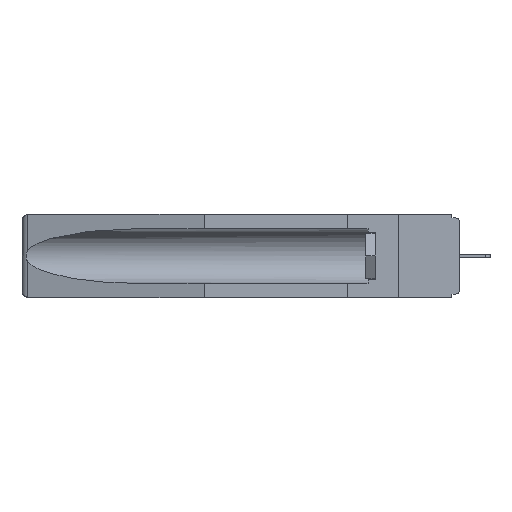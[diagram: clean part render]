
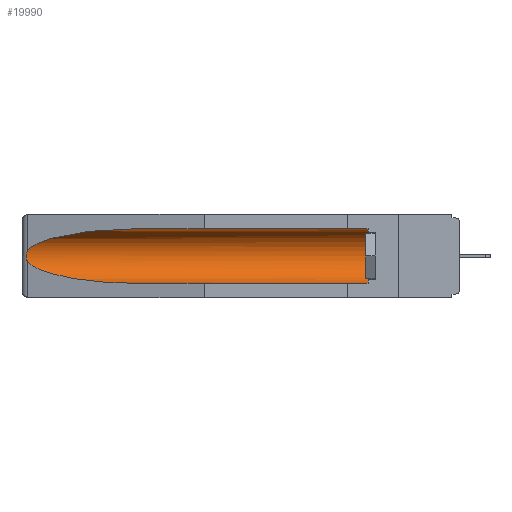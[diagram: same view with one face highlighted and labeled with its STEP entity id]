
A CAD part, left-side view. The second image highlights one B-rep face of the part: STEP entity #19990.
In plain terms, the highlighted cylindrical face has radius 2.857 mm (diameter 5.715 mm), a partial arc.
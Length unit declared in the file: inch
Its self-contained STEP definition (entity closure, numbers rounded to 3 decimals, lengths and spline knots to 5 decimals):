
#681 = CARTESIAN_POINT ( 'NONE',  ( 0.26654, 1.53092, -0.15636 ) ) ;
#915 = EDGE_LOOP ( 'NONE', ( #17573, #7100, #16528, #22189, #8965, #19200 ) ) ;
#920 = CARTESIAN_POINT ( 'NONE',  ( 0.26537, 1.52718, -0.19328 ) ) ;
#1057 = CARTESIAN_POINT ( 'NONE',  ( 0.26537, 1.52718, -0.14972 ) ) ;
#1384 = CARTESIAN_POINT ( 'NONE',  ( 0.155, -0.30754, -0.284 ) ) ;
#2085 = EDGE_CURVE ( 'NONE', #19488, #6543, #8350, .T. ) ;
#2313 = EDGE_CURVE ( 'NONE', #3320, #11349, #11604, .T. ) ;
#2711 = EDGE_CURVE ( 'NONE', #6543, #10084, #20772, .T. ) ;
#3014 = CARTESIAN_POINT ( 'NONE',  ( 0.26537, 1.52718, -0.14972 ) ) ;
#3318 = CARTESIAN_POINT ( 'NONE',  ( 0.155, -0.30754, -0.1715 ) ) ;
#3320 = VERTEX_POINT ( 'NONE', #4718 ) ;
#3870 = DIRECTION ( 'NONE',  ( 0., -1., 0. ) ) ;
#4206 = CARTESIAN_POINT ( 'NONE',  ( 0.21114, 1.30732, -0.059 ) ) ;
#4279 = VECTOR ( 'NONE', #20330, 39.37008 ) ;
#4718 = CARTESIAN_POINT ( 'NONE',  ( 0.155, 0.126, -0.284 ) ) ;
#4812 = CARTESIAN_POINT ( 'NONE',  ( 0.26537, 1.52718, -0.19328 ) ) ;
#4887 = EDGE_CURVE ( 'NONE', #3320, #6193, #9379, .T. ) ;
#6022 = CARTESIAN_POINT ( 'NONE',  ( 0.2673, 1.5327, -0.16383 ) ) ;
#6086 = CARTESIAN_POINT ( 'NONE',  ( 0.155, 1.07973, -0.284 ) ) ;
#6193 = VERTEX_POINT ( 'NONE', #15719 ) ;
#6500 = CARTESIAN_POINT ( 'NONE',  ( 0.26597, 1.52961, -0.15275 ) ) ;
#6543 = VERTEX_POINT ( 'NONE', #9733 ) ;
#6999 = LINE ( 'NONE', #14228, #7508 ) ;
#7100 = ORIENTED_EDGE ( 'NONE', *, *, #2711, .T. ) ;
#7508 = VECTOR ( 'NONE', #14156, 39.37008 ) ;
#7623 = EDGE_CURVE ( 'NONE', #10084, #11349, #15797, .T. ) ;
#8350 =( BOUNDED_CURVE ( )  B_SPLINE_CURVE ( 3, ( #16236, #4206, #19710, #1057 ),
 .UNSPECIFIED., .F., .T. ) 
 B_SPLINE_CURVE_WITH_KNOTS ( ( 4, 4 ),
 ( 4.71239, 6.08839 ),
 .UNSPECIFIED. ) 
 CURVE ( )  GEOMETRIC_REPRESENTATION_ITEM ( )  RATIONAL_B_SPLINE_CURVE ( ( 1., 0.848, 0.848, 1. ) ) 
 REPRESENTATION_ITEM ( '' )  );
#8965 = ORIENTED_EDGE ( 'NONE', *, *, #4887, .T. ) ;
#8966 = FACE_OUTER_BOUND ( 'NONE', #915, .T. ) ;
#9379 = CIRCLE ( 'NONE', #14799, 0.1125 ) ;
#9733 = CARTESIAN_POINT ( 'NONE',  ( 0.26537, 1.52718, -0.14972 ) ) ;
#10084 = VERTEX_POINT ( 'NONE', #920 ) ;
#10113 = CARTESIAN_POINT ( 'NONE',  ( 0.2673, 1.53269, -0.17917 ) ) ;
#10288 = CARTESIAN_POINT ( 'NONE',  ( 0.26597, 1.5296, -0.19026 ) ) ;
#10336 = EDGE_CURVE ( 'NONE', #6193, #19488, #6999, .T. ) ;
#10821 = DIRECTION ( 'NONE',  ( 0., 0., 1. ) ) ;
#11349 = VERTEX_POINT ( 'NONE', #12028 ) ;
#11463 = CARTESIAN_POINT ( 'NONE',  ( 0.25451, 1.48313, -0.24835 ) ) ;
#11604 = LINE ( 'NONE', #1384, #4279 ) ;
#12008 = DIRECTION ( 'NONE',  ( 0., 0., 1. ) ) ;
#12028 = CARTESIAN_POINT ( 'NONE',  ( 0.155, 1.07973, -0.284 ) ) ;
#12980 = CARTESIAN_POINT ( 'NONE',  ( 0.2675, 1.53308, -0.16763 ) ) ;
#13282 = CARTESIAN_POINT ( 'NONE',  ( 0.26537, 1.52718, -0.19328 ) ) ;
#14156 = DIRECTION ( 'NONE',  ( 0., 1., 0. ) ) ;
#14201 = CARTESIAN_POINT ( 'NONE',  ( 0.155, 0.126, -0.1715 ) ) ;
#14228 = CARTESIAN_POINT ( 'NONE',  ( 0.155, -0.30754, -0.059 ) ) ;
#14799 = AXIS2_PLACEMENT_3D ( 'NONE', #14201, #3870, #10821 ) ;
#14848 = CARTESIAN_POINT ( 'NONE',  ( 0.21114, 1.30732, -0.284 ) ) ;
#15719 = CARTESIAN_POINT ( 'NONE',  ( 0.155, 0.126, -0.059 ) ) ;
#15797 =( BOUNDED_CURVE ( )  B_SPLINE_CURVE ( 3, ( #13282, #11463, #14848, #6086 ),
 .UNSPECIFIED., .F., .F. ) 
 B_SPLINE_CURVE_WITH_KNOTS ( ( 4, 4 ),
 ( 0.1948, 1.5708 ),
 .UNSPECIFIED. ) 
 CURVE ( )  GEOMETRIC_REPRESENTATION_ITEM ( )  RATIONAL_B_SPLINE_CURVE ( ( 1., 0.848, 0.848, 1. ) ) 
 REPRESENTATION_ITEM ( '' )  );
#16236 = CARTESIAN_POINT ( 'NONE',  ( 0.155, 1.07973, -0.059 ) ) ;
#16528 = ORIENTED_EDGE ( 'NONE', *, *, #7623, .T. ) ;
#16928 = CARTESIAN_POINT ( 'NONE',  ( 0.26655, 1.53094, -0.18657 ) ) ;
#17573 = ORIENTED_EDGE ( 'NONE', *, *, #2085, .T. ) ;
#18430 = CYLINDRICAL_SURFACE ( 'NONE', #18681, 0.1125 ) ;
#18681 = AXIS2_PLACEMENT_3D ( 'NONE', #3318, #20769, #12008 ) ;
#19200 = ORIENTED_EDGE ( 'NONE', *, *, #10336, .T. ) ;
#19359 = CARTESIAN_POINT ( 'NONE',  ( 0.155, 1.07973, -0.059 ) ) ;
#19488 = VERTEX_POINT ( 'NONE', #19359 ) ;
#19710 = CARTESIAN_POINT ( 'NONE',  ( 0.25451, 1.48313, -0.09465 ) ) ;
#19990 = ADVANCED_FACE ( 'NONE', ( #8966 ), #18430, .F. ) ;
#20330 = DIRECTION ( 'NONE',  ( 0., 1., 0. ) ) ;
#20554 = CARTESIAN_POINT ( 'NONE',  ( 0.2675, 1.53308, -0.17534 ) ) ;
#20769 = DIRECTION ( 'NONE',  ( 0., 1., 0. ) ) ;
#20772 = B_SPLINE_CURVE_WITH_KNOTS ( 'NONE', 3,
 ( #3014, #6500, #681, #6022, #12980, #20554, #10113, #16928, #10288, #4812 ),
 .UNSPECIFIED., .F., .F.,
 ( 4, 2, 2, 2, 4 ),
 ( 0., 0.00029, 0.00058, 0.00087, 0.00117 ),
 .UNSPECIFIED. ) ;
#22189 = ORIENTED_EDGE ( 'NONE', *, *, #2313, .F. ) ;
